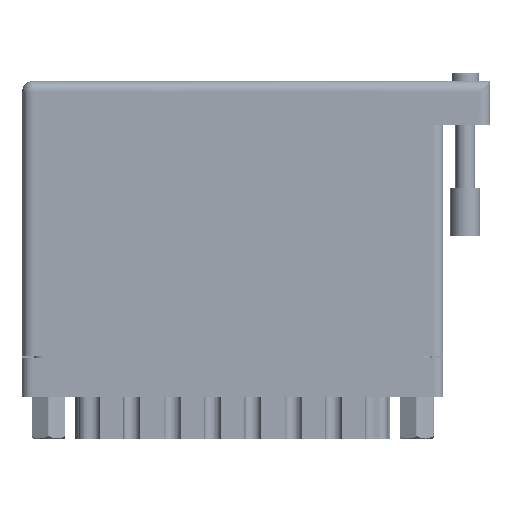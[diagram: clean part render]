
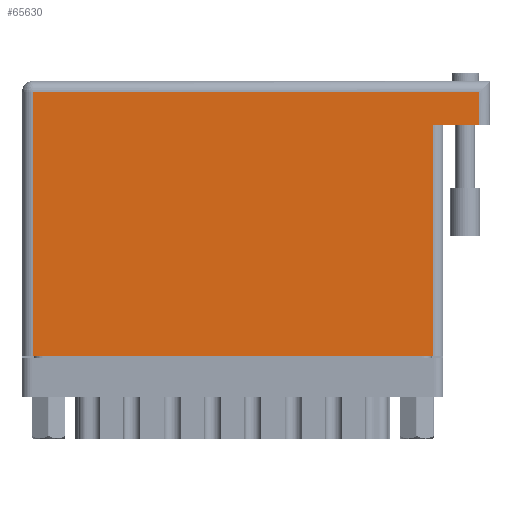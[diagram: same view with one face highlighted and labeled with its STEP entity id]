
A CAD part, front view. The second image highlights one B-rep face of the part: STEP entity #65630.
In plain terms, the highlighted face is planar.
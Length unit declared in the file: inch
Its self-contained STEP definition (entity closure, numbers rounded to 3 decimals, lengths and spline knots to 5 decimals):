
#145 = VERTEX_POINT ( 'NONE', #57363 ) ;
#1018 = PLANE ( 'NONE',  #27313 ) ;
#1446 = DIRECTION ( 'NONE',  ( -1., 0., 0. ) ) ;
#1691 = LINE ( 'NONE', #34256, #2354 ) ;
#2354 = VECTOR ( 'NONE', #48134, 39.37008 ) ;
#2651 = CARTESIAN_POINT ( 'NONE',  ( 0.07, 1.705, 0. ) ) ;
#3871 = ORIENTED_EDGE ( 'NONE', *, *, #58072, .T. ) ;
#7151 = CARTESIAN_POINT ( 'NONE',  ( 2.948, 1.495, 0. ) ) ;
#7436 = ORIENTED_EDGE ( 'NONE', *, *, #58108, .T. ) ;
#10221 = LINE ( 'NONE', #36715, #74693 ) ;
#10497 = ORIENTED_EDGE ( 'NONE', *, *, #31798, .T. ) ;
#13256 = LINE ( 'NONE', #23178, #42790 ) ;
#13652 = VECTOR ( 'NONE', #74422, 39.37008 ) ;
#19471 = DIRECTION ( 'NONE',  ( 0., 1., 0. ) ) ;
#23178 = CARTESIAN_POINT ( 'NONE',  ( 0.07, 0., 0. ) ) ;
#23959 = VERTEX_POINT ( 'NONE', #47790 ) ;
#24642 = VERTEX_POINT ( 'NONE', #77885 ) ;
#25662 = ORIENTED_EDGE ( 'NONE', *, *, #36785, .F. ) ;
#26855 = LINE ( 'NONE', #46431, #75146 ) ;
#27313 = AXIS2_PLACEMENT_3D ( 'NONE', #73978, #60932, #1446 ) ;
#31798 = EDGE_CURVE ( 'NONE', #56836, #24642, #13256, .T. ) ;
#34256 = CARTESIAN_POINT ( 'NONE',  ( 3.018, 1.495, 0. ) ) ;
#35699 = FACE_OUTER_BOUND ( 'NONE', #61879, .T. ) ;
#36437 = VERTEX_POINT ( 'NONE', #7151 ) ;
#36715 = CARTESIAN_POINT ( 'NONE',  ( 0., 1.705, 0. ) ) ;
#36785 = EDGE_CURVE ( 'NONE', #36437, #23959, #1691, .T. ) ;
#39882 = DIRECTION ( 'NONE',  ( 0., 1., 0. ) ) ;
#40403 = EDGE_CURVE ( 'NONE', #145, #56836, #10221, .T. ) ;
#41743 = LINE ( 'NONE', #79880, #77900 ) ;
#42790 = VECTOR ( 'NONE', #62297, 39.37008 ) ;
#46431 = CARTESIAN_POINT ( 'NONE',  ( 2.948, 1.775, 0. ) ) ;
#47514 = LINE ( 'NONE', #54027, #13652 ) ;
#47790 = CARTESIAN_POINT ( 'NONE',  ( 2.648, 1.495, 0. ) ) ;
#48134 = DIRECTION ( 'NONE',  ( -1., 0., 0. ) ) ;
#52566 = ORIENTED_EDGE ( 'NONE', *, *, #52886, .T. ) ;
#52886 = EDGE_CURVE ( 'NONE', #24642, #57403, #47514, .T. ) ;
#53197 = CARTESIAN_POINT ( 'NONE',  ( 2.648, 0., 0. ) ) ;
#54027 = CARTESIAN_POINT ( 'NONE',  ( 0., 0., 0. ) ) ;
#56836 = VERTEX_POINT ( 'NONE', #2651 ) ;
#57363 = CARTESIAN_POINT ( 'NONE',  ( 2.948, 1.705, 0. ) ) ;
#57403 = VERTEX_POINT ( 'NONE', #53197 ) ;
#58072 = EDGE_CURVE ( 'NONE', #57403, #23959, #41743, .T. ) ;
#58108 = EDGE_CURVE ( 'NONE', #36437, #145, #26855, .T. ) ;
#60932 = DIRECTION ( 'NONE',  ( 0., 0., -1. ) ) ;
#61879 = EDGE_LOOP ( 'NONE', ( #52566, #3871, #25662, #7436, #69764, #10497 ) ) ;
#62297 = DIRECTION ( 'NONE',  ( 0., -1., 0. ) ) ;
#63210 = DIRECTION ( 'NONE',  ( -1., 0., 0. ) ) ;
#65630 = ADVANCED_FACE ( 'NONE', ( #35699 ), #1018, .F. ) ;
#69764 = ORIENTED_EDGE ( 'NONE', *, *, #40403, .T. ) ;
#73978 = CARTESIAN_POINT ( 'NONE',  ( 0., 1.775, 0. ) ) ;
#74422 = DIRECTION ( 'NONE',  ( 1., 0., 0. ) ) ;
#74693 = VECTOR ( 'NONE', #63210, 39.37008 ) ;
#75146 = VECTOR ( 'NONE', #19471, 39.37008 ) ;
#77885 = CARTESIAN_POINT ( 'NONE',  ( 0.07, 0., 0. ) ) ;
#77900 = VECTOR ( 'NONE', #39882, 39.37008 ) ;
#79880 = CARTESIAN_POINT ( 'NONE',  ( 2.648, 1.495, 0. ) ) ;
